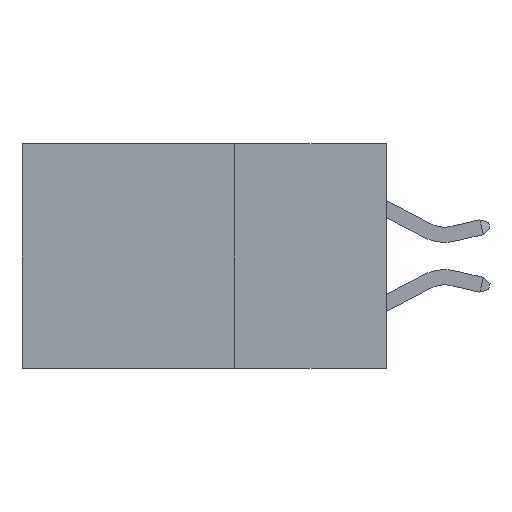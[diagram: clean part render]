
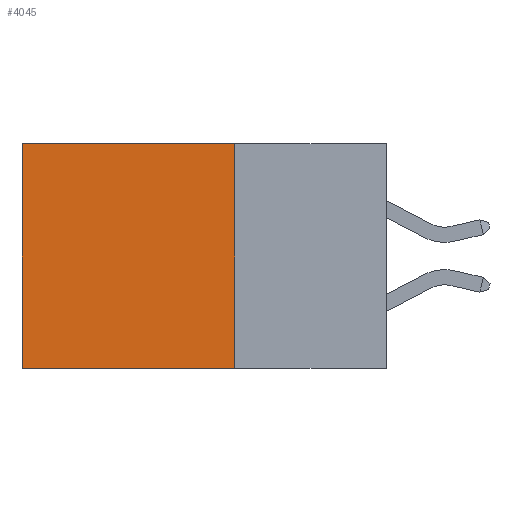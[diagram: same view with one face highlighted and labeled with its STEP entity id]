
A CAD part, left-side view. The second image highlights one B-rep face of the part: STEP entity #4045.
In plain terms, the highlighted planar face has unit normal (-1, 0, 0).
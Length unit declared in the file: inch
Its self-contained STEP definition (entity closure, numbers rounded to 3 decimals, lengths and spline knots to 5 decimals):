
#663 = ORIENTED_EDGE ( 'NONE', *, *, #9196, .F. ) ;
#711 = AXIS2_PLACEMENT_3D ( 'NONE', #10638, #10632, #9681 ) ;
#1130 = EDGE_LOOP ( 'NONE', ( #8319, #663, #5774, #10279 ) ) ;
#1306 = VERTEX_POINT ( 'NONE', #2389 ) ;
#1701 = CARTESIAN_POINT ( 'NONE',  ( 0.2615, 0.6, -0.37 ) ) ;
#1730 = VERTEX_POINT ( 'NONE', #4751 ) ;
#2389 = CARTESIAN_POINT ( 'NONE',  ( 0.2615, 0.6, -0.37 ) ) ;
#2562 = DIRECTION ( 'NONE',  ( 0., 1., 0. ) ) ;
#2661 = DIRECTION ( 'NONE',  ( 0., 0., -1. ) ) ;
#3863 = CARTESIAN_POINT ( 'NONE',  ( 0.2615, 0.25, 0. ) ) ;
#4045 = ADVANCED_FACE ( 'NONE', ( #6861 ), #10651, .F. ) ;
#4655 = VECTOR ( 'NONE', #5250, 39.37008 ) ;
#4751 = CARTESIAN_POINT ( 'NONE',  ( 0.2615, 0.25, -0.37 ) ) ;
#4842 = CARTESIAN_POINT ( 'NONE',  ( 0.2615, 0.6, 0. ) ) ;
#4951 = LINE ( 'NONE', #9058, #4655 ) ;
#5250 = DIRECTION ( 'NONE',  ( 0., 0., -1. ) ) ;
#5415 = EDGE_CURVE ( 'NONE', #11247, #1730, #4951, .T. ) ;
#5774 = ORIENTED_EDGE ( 'NONE', *, *, #5415, .F. ) ;
#6142 = VECTOR ( 'NONE', #10221, 39.37008 ) ;
#6861 = FACE_OUTER_BOUND ( 'NONE', #1130, .T. ) ;
#7607 = LINE ( 'NONE', #9842, #11777 ) ;
#8319 = ORIENTED_EDGE ( 'NONE', *, *, #9937, .T. ) ;
#8600 = LINE ( 'NONE', #3863, #6142 ) ;
#9058 = CARTESIAN_POINT ( 'NONE',  ( 0.2615, 0.25, -0.37 ) ) ;
#9179 = VECTOR ( 'NONE', #2661, 39.37008 ) ;
#9196 = EDGE_CURVE ( 'NONE', #1730, #1306, #7607, .T. ) ;
#9504 = CARTESIAN_POINT ( 'NONE',  ( 0.2615, 0.25, 0. ) ) ;
#9681 = DIRECTION ( 'NONE',  ( 0., 0., -1. ) ) ;
#9842 = CARTESIAN_POINT ( 'NONE',  ( 0.2615, 0.25, -0.37 ) ) ;
#9937 = EDGE_CURVE ( 'NONE', #10162, #1306, #11537, .T. ) ;
#10162 = VERTEX_POINT ( 'NONE', #4842 ) ;
#10221 = DIRECTION ( 'NONE',  ( 0., 1., 0. ) ) ;
#10279 = ORIENTED_EDGE ( 'NONE', *, *, #11703, .T. ) ;
#10632 = DIRECTION ( 'NONE',  ( 1., 0., 0. ) ) ;
#10638 = CARTESIAN_POINT ( 'NONE',  ( 0.2615, 0.25, -0.37 ) ) ;
#10651 = PLANE ( 'NONE',  #711 ) ;
#11247 = VERTEX_POINT ( 'NONE', #9504 ) ;
#11537 = LINE ( 'NONE', #1701, #9179 ) ;
#11703 = EDGE_CURVE ( 'NONE', #11247, #10162, #8600, .T. ) ;
#11777 = VECTOR ( 'NONE', #2562, 39.37008 ) ;
